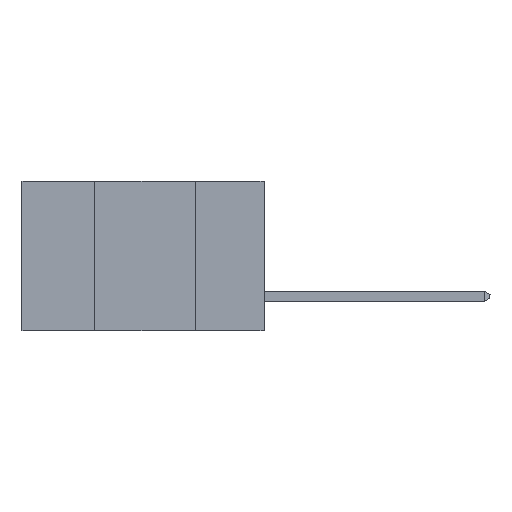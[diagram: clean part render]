
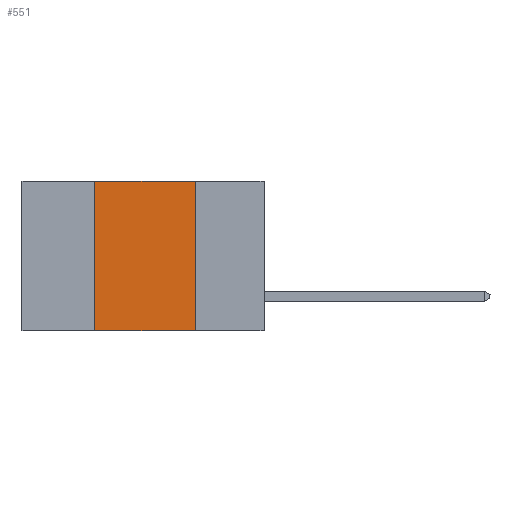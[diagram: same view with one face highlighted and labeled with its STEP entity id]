
A CAD part, left-side view. The second image highlights one B-rep face of the part: STEP entity #551.
In plain terms, the highlighted planar face has unit normal (-1, 0, 0).
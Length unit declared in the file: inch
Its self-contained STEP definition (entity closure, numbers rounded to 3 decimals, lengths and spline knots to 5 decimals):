
#269 = LINE ( 'NONE', #3071, #14895 ) ;
#551 = ADVANCED_FACE ( 'NONE', ( #24206 ), #10702, .F. ) ;
#1536 = VERTEX_POINT ( 'NONE', #24459 ) ;
#1895 = VECTOR ( 'NONE', #18680, 39.37008 ) ;
#2231 = VECTOR ( 'NONE', #19321, 39.37008 ) ;
#3071 = CARTESIAN_POINT ( 'NONE',  ( 0., 0.6, -0.37 ) ) ;
#3104 = EDGE_LOOP ( 'NONE', ( #24293, #7268, #17899, #7877 ) ) ;
#3738 = LINE ( 'NONE', #6894, #1895 ) ;
#4836 = EDGE_CURVE ( 'NONE', #21076, #8165, #3738, .T. ) ;
#6381 = LINE ( 'NONE', #19867, #20376 ) ;
#6523 = DIRECTION ( 'NONE',  ( 0., 0., -1. ) ) ;
#6712 = EDGE_CURVE ( 'NONE', #18056, #1536, #6381, .T. ) ;
#6894 = CARTESIAN_POINT ( 'NONE',  ( 0., 0.17, 0. ) ) ;
#7268 = ORIENTED_EDGE ( 'NONE', *, *, #11796, .F. ) ;
#7423 = LINE ( 'NONE', #9372, #2231 ) ;
#7877 = ORIENTED_EDGE ( 'NONE', *, *, #17322, .T. ) ;
#8165 = VERTEX_POINT ( 'NONE', #15472 ) ;
#9372 = CARTESIAN_POINT ( 'NONE',  ( 0., 0.6, 0. ) ) ;
#10702 = PLANE ( 'NONE',  #21827 ) ;
#11796 = EDGE_CURVE ( 'NONE', #1536, #21076, #7423, .T. ) ;
#11845 = CARTESIAN_POINT ( 'NONE',  ( 0., 0.42, -0.37 ) ) ;
#13123 = DIRECTION ( 'NONE',  ( 0., -1., 0. ) ) ;
#14895 = VECTOR ( 'NONE', #13123, 39.37008 ) ;
#15472 = CARTESIAN_POINT ( 'NONE',  ( 0., 0.17, -0.37 ) ) ;
#17322 = EDGE_CURVE ( 'NONE', #18056, #8165, #269, .T. ) ;
#17899 = ORIENTED_EDGE ( 'NONE', *, *, #6712, .F. ) ;
#18056 = VERTEX_POINT ( 'NONE', #11845 ) ;
#18205 = DIRECTION ( 'NONE',  ( 1., 0., 0. ) ) ;
#18680 = DIRECTION ( 'NONE',  ( 0., 0., -1. ) ) ;
#19321 = DIRECTION ( 'NONE',  ( 0., -1., 0. ) ) ;
#19867 = CARTESIAN_POINT ( 'NONE',  ( 0., 0.42, 0. ) ) ;
#20376 = VECTOR ( 'NONE', #21659, 39.37008 ) ;
#21076 = VERTEX_POINT ( 'NONE', #24166 ) ;
#21659 = DIRECTION ( 'NONE',  ( 0., 0., 1. ) ) ;
#21827 = AXIS2_PLACEMENT_3D ( 'NONE', #22262, #18205, #6523 ) ;
#22262 = CARTESIAN_POINT ( 'NONE',  ( 0., 0.6, 0. ) ) ;
#24166 = CARTESIAN_POINT ( 'NONE',  ( 0., 0.17, 0. ) ) ;
#24206 = FACE_OUTER_BOUND ( 'NONE', #3104, .T. ) ;
#24293 = ORIENTED_EDGE ( 'NONE', *, *, #4836, .F. ) ;
#24459 = CARTESIAN_POINT ( 'NONE',  ( 0., 0.42, 0. ) ) ;
